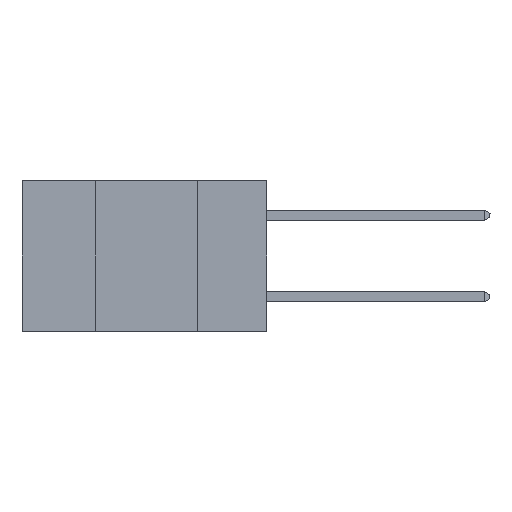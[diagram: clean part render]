
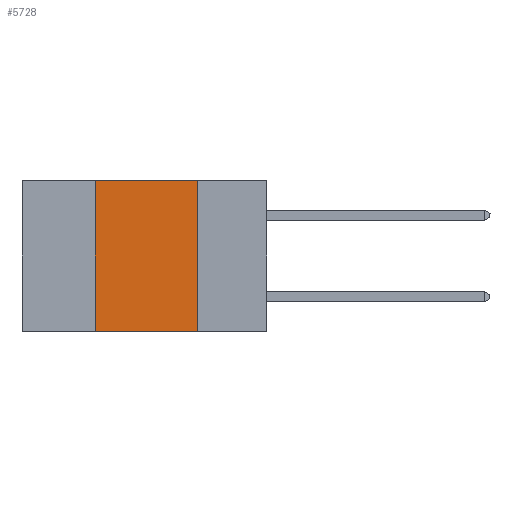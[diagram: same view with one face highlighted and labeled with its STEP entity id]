
A CAD part, left-side view. The second image highlights one B-rep face of the part: STEP entity #5728.
In plain terms, the highlighted planar face has unit normal (-1, 0, 0).
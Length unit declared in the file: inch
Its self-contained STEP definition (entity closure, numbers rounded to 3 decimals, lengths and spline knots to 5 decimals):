
#658 = CARTESIAN_POINT ( 'NONE',  ( 0., 0.17, -0.37 ) ) ;
#1234 = ORIENTED_EDGE ( 'NONE', *, *, #9450, .F. ) ;
#1240 = EDGE_LOOP ( 'NONE', ( #4735, #1234, #4238, #11320 ) ) ;
#1455 = DIRECTION ( 'NONE',  ( 0., 0., 1. ) ) ;
#1590 = LINE ( 'NONE', #2637, #13999 ) ;
#1635 = CARTESIAN_POINT ( 'NONE',  ( 0., 0.42, -0.37 ) ) ;
#1652 = FACE_OUTER_BOUND ( 'NONE', #1240, .T. ) ;
#2190 = VERTEX_POINT ( 'NONE', #3724 ) ;
#2209 = EDGE_CURVE ( 'NONE', #11446, #2190, #12789, .T. ) ;
#2637 = CARTESIAN_POINT ( 'NONE',  ( 0., 0.6, 0. ) ) ;
#3538 = CARTESIAN_POINT ( 'NONE',  ( 0., 0.17, 0. ) ) ;
#3724 = CARTESIAN_POINT ( 'NONE',  ( 0., 0.42, 0. ) ) ;
#3835 = CARTESIAN_POINT ( 'NONE',  ( 0., 0.6, -0.37 ) ) ;
#4238 = ORIENTED_EDGE ( 'NONE', *, *, #2209, .F. ) ;
#4735 = ORIENTED_EDGE ( 'NONE', *, *, #4855, .F. ) ;
#4855 = EDGE_CURVE ( 'NONE', #9667, #5269, #12607, .T. ) ;
#5083 = DIRECTION ( 'NONE',  ( 0., 0., -1. ) ) ;
#5199 = CARTESIAN_POINT ( 'NONE',  ( 0., 0.42, 0. ) ) ;
#5269 = VERTEX_POINT ( 'NONE', #658 ) ;
#5728 = ADVANCED_FACE ( 'NONE', ( #1652 ), #10232, .F. ) ;
#9164 = DIRECTION ( 'NONE',  ( 0., -1., 0. ) ) ;
#9166 = DIRECTION ( 'NONE',  ( 1., 0., 0. ) ) ;
#9450 = EDGE_CURVE ( 'NONE', #2190, #9667, #1590, .T. ) ;
#9667 = VERTEX_POINT ( 'NONE', #3538 ) ;
#10232 = PLANE ( 'NONE',  #13552 ) ;
#10799 = VECTOR ( 'NONE', #5083, 39.37008 ) ;
#10853 = VECTOR ( 'NONE', #9164, 39.37008 ) ;
#11075 = EDGE_CURVE ( 'NONE', #11446, #5269, #12574, .T. ) ;
#11320 = ORIENTED_EDGE ( 'NONE', *, *, #11075, .T. ) ;
#11403 = CARTESIAN_POINT ( 'NONE',  ( 0., 0.17, 0. ) ) ;
#11440 = CARTESIAN_POINT ( 'NONE',  ( 0., 0.6, 0. ) ) ;
#11446 = VERTEX_POINT ( 'NONE', #1635 ) ;
#11506 = DIRECTION ( 'NONE',  ( 0., 0., -1. ) ) ;
#12452 = DIRECTION ( 'NONE',  ( 0., -1., 0. ) ) ;
#12574 = LINE ( 'NONE', #3835, #10853 ) ;
#12607 = LINE ( 'NONE', #11403, #10799 ) ;
#12789 = LINE ( 'NONE', #5199, #13048 ) ;
#13048 = VECTOR ( 'NONE', #1455, 39.37008 ) ;
#13552 = AXIS2_PLACEMENT_3D ( 'NONE', #11440, #9166, #11506 ) ;
#13999 = VECTOR ( 'NONE', #12452, 39.37008 ) ;
